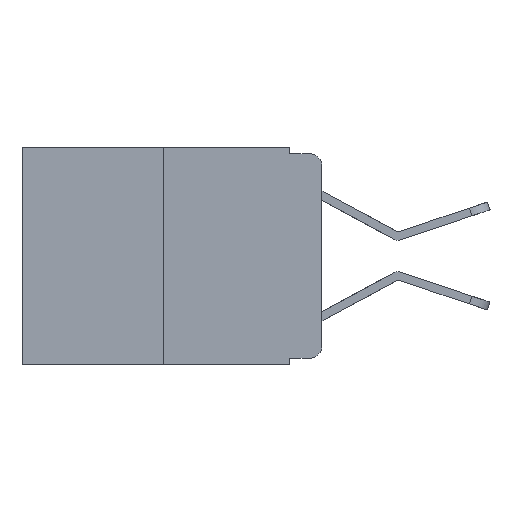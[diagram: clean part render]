
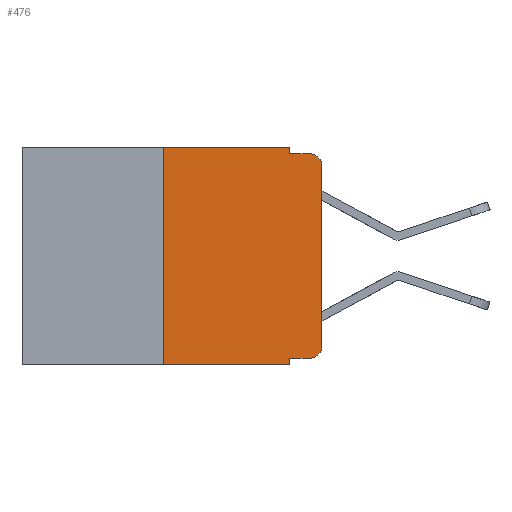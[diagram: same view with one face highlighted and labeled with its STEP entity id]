
A CAD part, left-side view. The second image highlights one B-rep face of the part: STEP entity #476.
In plain terms, the highlighted planar face has unit normal (-1, 0, 0).
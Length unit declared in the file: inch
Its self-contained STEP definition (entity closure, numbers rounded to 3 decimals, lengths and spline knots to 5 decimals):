
#96 = DIRECTION ( 'NONE',  ( 0., 0., 1. ) ) ;
#314 = VECTOR ( 'NONE', #6046, 39.37008 ) ;
#476 = ADVANCED_FACE ( 'NONE', ( #4043 ), #9174, .F. ) ;
#626 = ORIENTED_EDGE ( 'NONE', *, *, #8614, .F. ) ;
#787 = LINE ( 'NONE', #5887, #11164 ) ;
#996 = LINE ( 'NONE', #4242, #11300 ) ;
#1058 = ORIENTED_EDGE ( 'NONE', *, *, #8010, .T. ) ;
#1091 = EDGE_CURVE ( 'NONE', #8519, #11533, #10594, .T. ) ;
#1370 = DIRECTION ( 'NONE',  ( 0., -1., 0. ) ) ;
#1780 = VECTOR ( 'NONE', #8682, 39.37008 ) ;
#2055 = ORIENTED_EDGE ( 'NONE', *, *, #10965, .T. ) ;
#2159 = DIRECTION ( 'NONE',  ( 0., 0., -1. ) ) ;
#2439 = ORIENTED_EDGE ( 'NONE', *, *, #9778, .F. ) ;
#2881 = VERTEX_POINT ( 'NONE', #12187 ) ;
#2882 = CARTESIAN_POINT ( 'NONE',  ( 0., 0.051, -0.01 ) ) ;
#3271 = LINE ( 'NONE', #10422, #3633 ) ;
#3486 = CIRCLE ( 'NONE', #6621, 0.02 ) ;
#3633 = VECTOR ( 'NONE', #10465, 39.37008 ) ;
#3646 = LINE ( 'NONE', #2882, #314 ) ;
#4043 = FACE_OUTER_BOUND ( 'NONE', #12654, .T. ) ;
#4242 = CARTESIAN_POINT ( 'NONE',  ( 0., 0.051, 0. ) ) ;
#4483 = DIRECTION ( 'NONE',  ( -1., 0., 0. ) ) ;
#4874 = CARTESIAN_POINT ( 'NONE',  ( 0., 0.473, 0. ) ) ;
#5032 = CARTESIAN_POINT ( 'NONE',  ( 0., 0.473, -0.343 ) ) ;
#5249 = VERTEX_POINT ( 'NONE', #11332 ) ;
#5625 = VERTEX_POINT ( 'NONE', #8545 ) ;
#5885 = CIRCLE ( 'NONE', #9039, 0.02 ) ;
#5887 = CARTESIAN_POINT ( 'NONE',  ( 0., 0.25, 0. ) ) ;
#6046 = DIRECTION ( 'NONE',  ( 0., -1., 0. ) ) ;
#6325 = CARTESIAN_POINT ( 'NONE',  ( 0., 0.02, -0.313 ) ) ;
#6621 = AXIS2_PLACEMENT_3D ( 'NONE', #6325, #12668, #7297 ) ;
#6781 = CARTESIAN_POINT ( 'NONE',  ( 0., 0.473, 0. ) ) ;
#6833 = CARTESIAN_POINT ( 'NONE',  ( 0., 0.051, -0.343 ) ) ;
#7038 = VERTEX_POINT ( 'NONE', #11613 ) ;
#7297 = DIRECTION ( 'NONE',  ( 0., 0., -1. ) ) ;
#7396 = EDGE_CURVE ( 'NONE', #2881, #5625, #3486, .T. ) ;
#7764 = CARTESIAN_POINT ( 'NONE',  ( 0., 0.051, -0.333 ) ) ;
#7989 = VECTOR ( 'NONE', #2159, 39.37008 ) ;
#8010 = EDGE_CURVE ( 'NONE', #5249, #2881, #10044, .T. ) ;
#8040 = VERTEX_POINT ( 'NONE', #12198 ) ;
#8163 = ORIENTED_EDGE ( 'NONE', *, *, #9221, .F. ) ;
#8288 = CARTESIAN_POINT ( 'NONE',  ( 0., 0.051, 0. ) ) ;
#8519 = VERTEX_POINT ( 'NONE', #12657 ) ;
#8545 = CARTESIAN_POINT ( 'NONE',  ( 0., 0., -0.313 ) ) ;
#8614 = EDGE_CURVE ( 'NONE', #5249, #11533, #9775, .T. ) ;
#8682 = DIRECTION ( 'NONE',  ( 0., -1., 0. ) ) ;
#8727 = ORIENTED_EDGE ( 'NONE', *, *, #1091, .T. ) ;
#9039 = AXIS2_PLACEMENT_3D ( 'NONE', #10085, #4483, #10960 ) ;
#9125 = LINE ( 'NONE', #4874, #11452 ) ;
#9163 = EDGE_CURVE ( 'NONE', #10591, #8040, #9125, .T. ) ;
#9174 = PLANE ( 'NONE',  #10042 ) ;
#9220 = DIRECTION ( 'NONE',  ( 1., 0., 0. ) ) ;
#9221 = EDGE_CURVE ( 'NONE', #8519, #10591, #787, .T. ) ;
#9286 = ORIENTED_EDGE ( 'NONE', *, *, #7396, .T. ) ;
#9309 = VERTEX_POINT ( 'NONE', #9604 ) ;
#9407 = ORIENTED_EDGE ( 'NONE', *, *, #11571, .T. ) ;
#9604 = CARTESIAN_POINT ( 'NONE',  ( 0., 0.051, -0.01 ) ) ;
#9775 = LINE ( 'NONE', #8288, #7989 ) ;
#9778 = EDGE_CURVE ( 'NONE', #8040, #9309, #996, .T. ) ;
#10042 = AXIS2_PLACEMENT_3D ( 'NONE', #6781, #9220, #12991 ) ;
#10044 = LINE ( 'NONE', #7764, #1780 ) ;
#10085 = CARTESIAN_POINT ( 'NONE',  ( 0., 0.02, -0.03 ) ) ;
#10237 = ORIENTED_EDGE ( 'NONE', *, *, #9163, .F. ) ;
#10384 = EDGE_CURVE ( 'NONE', #9309, #7038, #3646, .T. ) ;
#10422 = CARTESIAN_POINT ( 'NONE',  ( 0., 0., 0. ) ) ;
#10465 = DIRECTION ( 'NONE',  ( 0., 0., 1. ) ) ;
#10591 = VERTEX_POINT ( 'NONE', #11597 ) ;
#10594 = LINE ( 'NONE', #5032, #12994 ) ;
#10960 = DIRECTION ( 'NONE',  ( 0., 0., -1. ) ) ;
#10965 = EDGE_CURVE ( 'NONE', #11933, #7038, #5885, .T. ) ;
#11164 = VECTOR ( 'NONE', #96, 39.37008 ) ;
#11300 = VECTOR ( 'NONE', #12607, 39.37008 ) ;
#11332 = CARTESIAN_POINT ( 'NONE',  ( 0., 0.051, -0.333 ) ) ;
#11452 = VECTOR ( 'NONE', #1370, 39.37008 ) ;
#11533 = VERTEX_POINT ( 'NONE', #6833 ) ;
#11571 = EDGE_CURVE ( 'NONE', #5625, #11933, #3271, .T. ) ;
#11597 = CARTESIAN_POINT ( 'NONE',  ( 0., 0.25, 0. ) ) ;
#11613 = CARTESIAN_POINT ( 'NONE',  ( 0., 0.02, -0.01 ) ) ;
#11933 = VERTEX_POINT ( 'NONE', #12635 ) ;
#12039 = DIRECTION ( 'NONE',  ( 0., -1., 0. ) ) ;
#12187 = CARTESIAN_POINT ( 'NONE',  ( 0., 0.02, -0.333 ) ) ;
#12198 = CARTESIAN_POINT ( 'NONE',  ( 0., 0.051, 0. ) ) ;
#12336 = ORIENTED_EDGE ( 'NONE', *, *, #10384, .F. ) ;
#12607 = DIRECTION ( 'NONE',  ( 0., 0., -1. ) ) ;
#12635 = CARTESIAN_POINT ( 'NONE',  ( 0., 0., -0.03 ) ) ;
#12654 = EDGE_LOOP ( 'NONE', ( #9407, #2055, #12336, #2439, #10237, #8163, #8727, #626, #1058, #9286 ) ) ;
#12657 = CARTESIAN_POINT ( 'NONE',  ( 0., 0.25, -0.343 ) ) ;
#12668 = DIRECTION ( 'NONE',  ( -1., 0., 0. ) ) ;
#12991 = DIRECTION ( 'NONE',  ( 0., 0., -1. ) ) ;
#12994 = VECTOR ( 'NONE', #12039, 39.37008 ) ;
